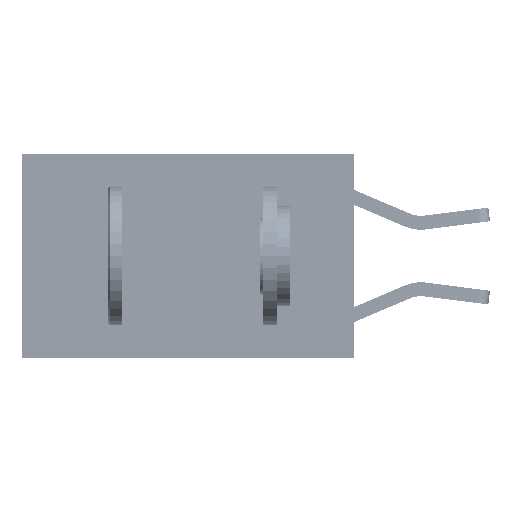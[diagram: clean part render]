
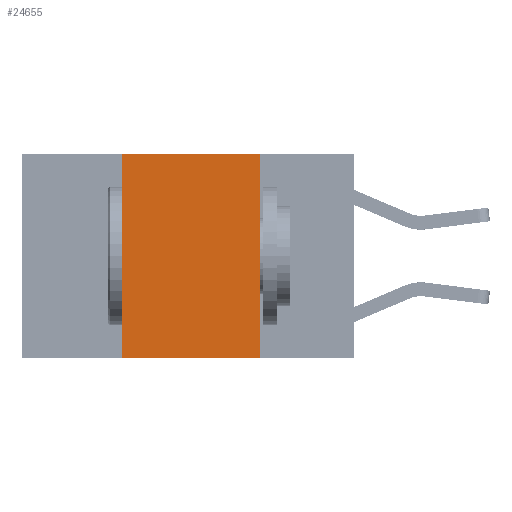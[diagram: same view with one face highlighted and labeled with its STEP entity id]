
A CAD part, left-side view. The second image highlights one B-rep face of the part: STEP entity #24655.
In plain terms, the highlighted planar face has unit normal (-1, 0, 0).
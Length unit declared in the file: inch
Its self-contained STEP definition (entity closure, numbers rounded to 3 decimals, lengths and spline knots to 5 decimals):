
#5 = FACE_OUTER_BOUND ( 'NONE', #17839, .T. ) ;
#313 = EDGE_CURVE ( 'NONE', #25063, #11225, #31487, .T. ) ;
#885 = ORIENTED_EDGE ( 'NONE', *, *, #313, .F. ) ;
#4003 = CARTESIAN_POINT ( 'NONE',  ( 0., 0.42, 0. ) ) ;
#5305 = CARTESIAN_POINT ( 'NONE',  ( 0., 0.17, -0.37 ) ) ;
#5367 = PLANE ( 'NONE',  #7128 ) ;
#6583 = VERTEX_POINT ( 'NONE', #26611 ) ;
#7128 = AXIS2_PLACEMENT_3D ( 'NONE', #12911, #30877, #7882 ) ;
#7165 = ORIENTED_EDGE ( 'NONE', *, *, #33043, .F. ) ;
#7882 = DIRECTION ( 'NONE',  ( 0., 0., -1. ) ) ;
#8335 = CARTESIAN_POINT ( 'NONE',  ( 0., 0.17, 0. ) ) ;
#8336 = CARTESIAN_POINT ( 'NONE',  ( 0., 0.17, 0. ) ) ;
#9054 = VERTEX_POINT ( 'NONE', #23120 ) ;
#11225 = VERTEX_POINT ( 'NONE', #5305 ) ;
#12584 = VECTOR ( 'NONE', #18941, 39.37008 ) ;
#12680 = EDGE_CURVE ( 'NONE', #9054, #11225, #12855, .T. ) ;
#12855 = LINE ( 'NONE', #18051, #28458 ) ;
#12911 = CARTESIAN_POINT ( 'NONE',  ( 0., 0.6, 0. ) ) ;
#16886 = VECTOR ( 'NONE', #27949, 39.37008 ) ;
#17839 = EDGE_LOOP ( 'NONE', ( #885, #7165, #30047, #24330 ) ) ;
#18051 = CARTESIAN_POINT ( 'NONE',  ( 0., 0.6, -0.37 ) ) ;
#18941 = DIRECTION ( 'NONE',  ( 0., 0., 1. ) ) ;
#19901 = VECTOR ( 'NONE', #23297, 39.37008 ) ;
#22770 = DIRECTION ( 'NONE',  ( 0., -1., 0. ) ) ;
#23120 = CARTESIAN_POINT ( 'NONE',  ( 0., 0.42, -0.37 ) ) ;
#23263 = CARTESIAN_POINT ( 'NONE',  ( 0., 0.6, 0. ) ) ;
#23297 = DIRECTION ( 'NONE',  ( 0., 0., -1. ) ) ;
#23829 = LINE ( 'NONE', #4003, #12584 ) ;
#24330 = ORIENTED_EDGE ( 'NONE', *, *, #12680, .T. ) ;
#24655 = ADVANCED_FACE ( 'NONE', ( #5 ), #5367, .F. ) ;
#25063 = VERTEX_POINT ( 'NONE', #8336 ) ;
#25938 = LINE ( 'NONE', #23263, #16886 ) ;
#26611 = CARTESIAN_POINT ( 'NONE',  ( 0., 0.42, 0. ) ) ;
#27949 = DIRECTION ( 'NONE',  ( 0., -1., 0. ) ) ;
#28458 = VECTOR ( 'NONE', #22770, 39.37008 ) ;
#30047 = ORIENTED_EDGE ( 'NONE', *, *, #32398, .F. ) ;
#30877 = DIRECTION ( 'NONE',  ( 1., 0., 0. ) ) ;
#31487 = LINE ( 'NONE', #8335, #19901 ) ;
#32398 = EDGE_CURVE ( 'NONE', #9054, #6583, #23829, .T. ) ;
#33043 = EDGE_CURVE ( 'NONE', #6583, #25063, #25938, .T. ) ;
